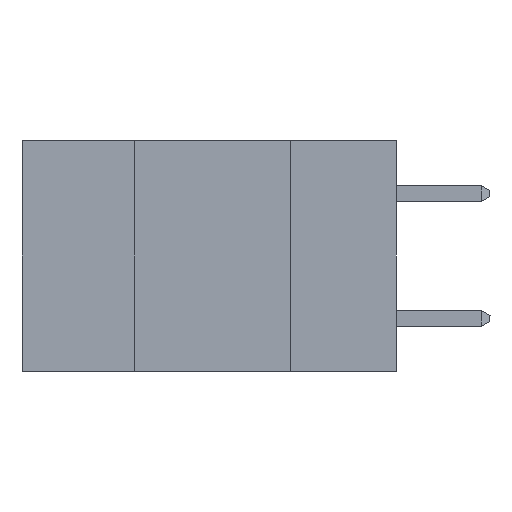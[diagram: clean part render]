
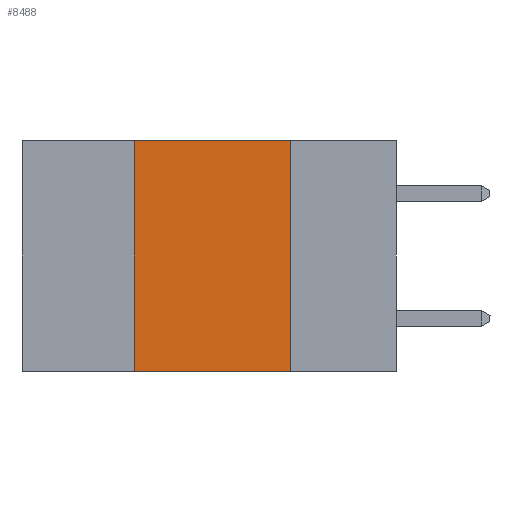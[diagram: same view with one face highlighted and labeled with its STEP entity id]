
A CAD part, left-side view. The second image highlights one B-rep face of the part: STEP entity #8488.
In plain terms, the highlighted planar face has unit normal (-1, 0, 0).
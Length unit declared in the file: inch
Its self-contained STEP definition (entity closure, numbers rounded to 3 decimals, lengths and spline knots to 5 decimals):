
#611 = CARTESIAN_POINT ( 'NONE',  ( 0., 0.17, -0.37 ) ) ;
#694 = DIRECTION ( 'NONE',  ( 0., 0., -1. ) ) ;
#747 = LINE ( 'NONE', #14586, #3534 ) ;
#974 = CARTESIAN_POINT ( 'NONE',  ( 0., 0.17, -0.37 ) ) ;
#1157 = VERTEX_POINT ( 'NONE', #3839 ) ;
#1630 = DIRECTION ( 'NONE',  ( 0., 0., -1. ) ) ;
#1668 = DIRECTION ( 'NONE',  ( 1., 0., 0. ) ) ;
#1673 = PLANE ( 'NONE',  #11499 ) ;
#1719 = CARTESIAN_POINT ( 'NONE',  ( 0., 0.6, 0. ) ) ;
#1721 = EDGE_CURVE ( 'NONE', #3684, #1157, #6132, .T. ) ;
#2669 = EDGE_CURVE ( 'NONE', #1157, #12763, #747, .T. ) ;
#2681 = VECTOR ( 'NONE', #11737, 39.37008 ) ;
#2884 = EDGE_LOOP ( 'NONE', ( #11018, #5402, #6736, #9080 ) ) ;
#3534 = VECTOR ( 'NONE', #14467, 39.37008 ) ;
#3595 = EDGE_CURVE ( 'NONE', #12763, #8607, #7735, .T. ) ;
#3684 = VERTEX_POINT ( 'NONE', #11720 ) ;
#3839 = CARTESIAN_POINT ( 'NONE',  ( 0., 0.42, 0. ) ) ;
#5402 = ORIENTED_EDGE ( 'NONE', *, *, #2669, .F. ) ;
#5877 = FACE_OUTER_BOUND ( 'NONE', #2884, .T. ) ;
#6132 = LINE ( 'NONE', #12605, #2681 ) ;
#6699 = VECTOR ( 'NONE', #9478, 39.37008 ) ;
#6736 = ORIENTED_EDGE ( 'NONE', *, *, #1721, .F. ) ;
#7735 = LINE ( 'NONE', #611, #14489 ) ;
#8461 = CARTESIAN_POINT ( 'NONE',  ( 0., 0.6, -0.37 ) ) ;
#8488 = ADVANCED_FACE ( 'NONE', ( #5877 ), #1673, .F. ) ;
#8607 = VERTEX_POINT ( 'NONE', #974 ) ;
#9080 = ORIENTED_EDGE ( 'NONE', *, *, #16547, .T. ) ;
#9478 = DIRECTION ( 'NONE',  ( 0., -1., 0. ) ) ;
#11018 = ORIENTED_EDGE ( 'NONE', *, *, #3595, .F. ) ;
#11499 = AXIS2_PLACEMENT_3D ( 'NONE', #1719, #1668, #1630 ) ;
#11720 = CARTESIAN_POINT ( 'NONE',  ( 0., 0.42, -0.37 ) ) ;
#11737 = DIRECTION ( 'NONE',  ( 0., 0., 1. ) ) ;
#12605 = CARTESIAN_POINT ( 'NONE',  ( 0., 0.42, -0.37 ) ) ;
#12763 = VERTEX_POINT ( 'NONE', #15733 ) ;
#13091 = LINE ( 'NONE', #8461, #6699 ) ;
#14467 = DIRECTION ( 'NONE',  ( 0., -1., 0. ) ) ;
#14489 = VECTOR ( 'NONE', #694, 39.37008 ) ;
#14586 = CARTESIAN_POINT ( 'NONE',  ( 0., 0.6, 0. ) ) ;
#15733 = CARTESIAN_POINT ( 'NONE',  ( 0., 0.17, 0. ) ) ;
#16547 = EDGE_CURVE ( 'NONE', #3684, #8607, #13091, .T. ) ;
